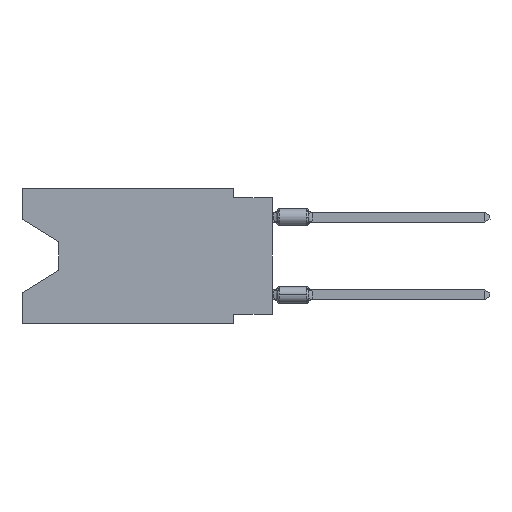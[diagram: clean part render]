
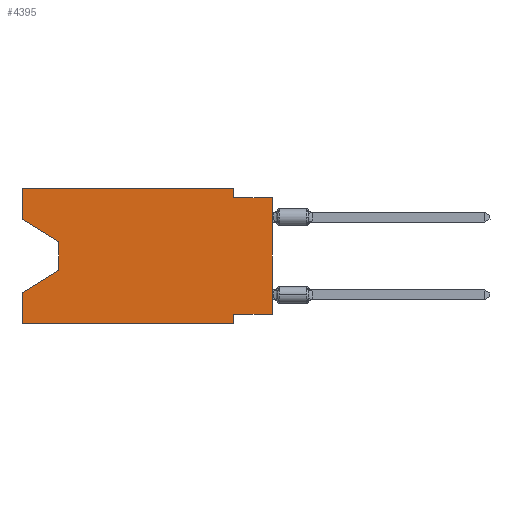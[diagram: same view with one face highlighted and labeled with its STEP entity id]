
A CAD part, left-side view. The second image highlights one B-rep face of the part: STEP entity #4395.
In plain terms, the highlighted planar face has unit normal (-1, 0, 0).
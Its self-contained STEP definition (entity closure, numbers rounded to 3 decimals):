
#636 = CARTESIAN_POINT ( 'NONE',  ( 0., 16.383, 0. ) ) ;
#758 = VERTEX_POINT ( 'NONE', #8095 ) ;
#846 = ORIENTED_EDGE ( 'NONE', *, *, #6919, .T. ) ;
#1065 = DIRECTION ( 'NONE',  ( 0., 0., -1. ) ) ;
#1217 = DIRECTION ( 'NONE',  ( 0., -0.855, -0.519 ) ) ;
#1262 = ORIENTED_EDGE ( 'NONE', *, *, #19110, .F. ) ;
#1602 = CARTESIAN_POINT ( 'NONE',  ( 0., 0., 0. ) ) ;
#1661 = ORIENTED_EDGE ( 'NONE', *, *, #12920, .F. ) ;
#2120 = DIRECTION ( 'NONE',  ( 0., -1., 0. ) ) ;
#2260 = CARTESIAN_POINT ( 'NONE',  ( 0., 2.54, 0. ) ) ;
#3335 = LINE ( 'NONE', #3458, #5462 ) ;
#3458 = CARTESIAN_POINT ( 'NONE',  ( 0., 16.383, 0. ) ) ;
#3691 = CARTESIAN_POINT ( 'NONE',  ( 0., 16.383, 0. ) ) ;
#3727 = LINE ( 'NONE', #21717, #14031 ) ;
#4017 = CARTESIAN_POINT ( 'NONE',  ( 0., 2.54, 0. ) ) ;
#4060 = CARTESIAN_POINT ( 'NONE',  ( 0., 16.383, 0. ) ) ;
#4395 = ADVANCED_FACE ( 'NONE', ( #16853 ), #10166, .F. ) ;
#4609 = EDGE_CURVE ( 'NONE', #20046, #12126, #15440, .T. ) ;
#4784 = CARTESIAN_POINT ( 'NONE',  ( 0., 2.54, -0.635 ) ) ;
#5031 = ORIENTED_EDGE ( 'NONE', *, *, #14738, .F. ) ;
#5048 = ORIENTED_EDGE ( 'NONE', *, *, #17432, .T. ) ;
#5152 = VERTEX_POINT ( 'NONE', #20845 ) ;
#5462 = VECTOR ( 'NONE', #10371, 1000. ) ;
#5563 = LINE ( 'NONE', #4060, #11293 ) ;
#5723 = EDGE_CURVE ( 'NONE', #17282, #21972, #11403, .T. ) ;
#5893 = LINE ( 'NONE', #12917, #9303 ) ;
#6027 = VECTOR ( 'NONE', #17652, 1000. ) ;
#6534 = VERTEX_POINT ( 'NONE', #636 ) ;
#6652 = CARTESIAN_POINT ( 'NONE',  ( 0., 0., -0.635 ) ) ;
#6772 = VECTOR ( 'NONE', #22127, 1000. ) ;
#6839 = CARTESIAN_POINT ( 'NONE',  ( 0., 16.383, -8.89 ) ) ;
#6886 = ORIENTED_EDGE ( 'NONE', *, *, #7499, .F. ) ;
#6919 = EDGE_CURVE ( 'NONE', #21859, #15292, #5893, .T. ) ;
#7285 = DIRECTION ( 'NONE',  ( 0., 0., -1. ) ) ;
#7499 = EDGE_CURVE ( 'NONE', #17193, #758, #7719, .T. ) ;
#7719 = LINE ( 'NONE', #6652, #15953 ) ;
#8095 = CARTESIAN_POINT ( 'NONE',  ( 0., 0., -0.635 ) ) ;
#8493 = DIRECTION ( 'NONE',  ( 0., -1., 0. ) ) ;
#8780 = CARTESIAN_POINT ( 'NONE',  ( 0., 16.383, -6.852 ) ) ;
#8879 = ORIENTED_EDGE ( 'NONE', *, *, #4609, .F. ) ;
#9303 = VECTOR ( 'NONE', #17780, 1000. ) ;
#9348 = LINE ( 'NONE', #11080, #10402 ) ;
#9779 = CARTESIAN_POINT ( 'NONE',  ( 0., 0., -8.255 ) ) ;
#10044 = DIRECTION ( 'NONE',  ( 1., 0., 0. ) ) ;
#10166 = PLANE ( 'NONE',  #11913 ) ;
#10371 = DIRECTION ( 'NONE',  ( 0., 0., 1. ) ) ;
#10402 = VECTOR ( 'NONE', #7285, 1000. ) ;
#10434 = LINE ( 'NONE', #15752, #20617 ) ;
#10548 = VECTOR ( 'NONE', #14482, 1000. ) ;
#11080 = CARTESIAN_POINT ( 'NONE',  ( 0., 2.54, -8.89 ) ) ;
#11215 = EDGE_CURVE ( 'NONE', #6534, #16757, #5563, .T. ) ;
#11293 = VECTOR ( 'NONE', #2120, 1000. ) ;
#11342 = ORIENTED_EDGE ( 'NONE', *, *, #14582, .T. ) ;
#11403 = LINE ( 'NONE', #16375, #13415 ) ;
#11913 = AXIS2_PLACEMENT_3D ( 'NONE', #18822, #10044, #1065 ) ;
#12126 = VERTEX_POINT ( 'NONE', #21549 ) ;
#12835 = CARTESIAN_POINT ( 'NONE',  ( 0., 0., -8.255 ) ) ;
#12917 = CARTESIAN_POINT ( 'NONE',  ( 0., 16.383, -8.89 ) ) ;
#12920 = EDGE_CURVE ( 'NONE', #5152, #6534, #3335, .T. ) ;
#13415 = VECTOR ( 'NONE', #21563, 1000. ) ;
#13595 = CARTESIAN_POINT ( 'NONE',  ( 0., 13.97, -3.505 ) ) ;
#13716 = EDGE_CURVE ( 'NONE', #5152, #14008, #10434, .T. ) ;
#14008 = VERTEX_POINT ( 'NONE', #13595 ) ;
#14031 = VECTOR ( 'NONE', #18141, 1000. ) ;
#14302 = LINE ( 'NONE', #3691, #6027 ) ;
#14482 = DIRECTION ( 'NONE',  ( 0., 0., -1. ) ) ;
#14582 = EDGE_CURVE ( 'NONE', #20046, #758, #17387, .T. ) ;
#14738 = EDGE_CURVE ( 'NONE', #16757, #17193, #18050, .T. ) ;
#14981 = ORIENTED_EDGE ( 'NONE', *, *, #11215, .F. ) ;
#15292 = VERTEX_POINT ( 'NONE', #21714 ) ;
#15440 = LINE ( 'NONE', #9779, #6772 ) ;
#15671 = DIRECTION ( 'NONE',  ( 0., 0., 1. ) ) ;
#15752 = CARTESIAN_POINT ( 'NONE',  ( 0., 16.383, -2.038 ) ) ;
#15953 = VECTOR ( 'NONE', #8493, 1000. ) ;
#16375 = CARTESIAN_POINT ( 'NONE',  ( 0., 13.97, -5.385 ) ) ;
#16757 = VERTEX_POINT ( 'NONE', #4017 ) ;
#16853 = FACE_OUTER_BOUND ( 'NONE', #22522, .T. ) ;
#17193 = VERTEX_POINT ( 'NONE', #4784 ) ;
#17282 = VERTEX_POINT ( 'NONE', #22096 ) ;
#17338 = ORIENTED_EDGE ( 'NONE', *, *, #20772, .F. ) ;
#17387 = LINE ( 'NONE', #1602, #19027 ) ;
#17432 = EDGE_CURVE ( 'NONE', #14008, #17282, #3727, .T. ) ;
#17652 = DIRECTION ( 'NONE',  ( 0., 0., 1. ) ) ;
#17780 = DIRECTION ( 'NONE',  ( 0., -1., 0. ) ) ;
#18050 = LINE ( 'NONE', #2260, #10548 ) ;
#18141 = DIRECTION ( 'NONE',  ( 0., 0., -1. ) ) ;
#18333 = ORIENTED_EDGE ( 'NONE', *, *, #5723, .T. ) ;
#18822 = CARTESIAN_POINT ( 'NONE',  ( 0., 16.383, 0. ) ) ;
#19027 = VECTOR ( 'NONE', #15671, 1000. ) ;
#19110 = EDGE_CURVE ( 'NONE', #12126, #15292, #9348, .T. ) ;
#20046 = VERTEX_POINT ( 'NONE', #12835 ) ;
#20267 = ORIENTED_EDGE ( 'NONE', *, *, #13716, .T. ) ;
#20617 = VECTOR ( 'NONE', #1217, 1000. ) ;
#20772 = EDGE_CURVE ( 'NONE', #21859, #21972, #14302, .T. ) ;
#20845 = CARTESIAN_POINT ( 'NONE',  ( 0., 16.383, -2.038 ) ) ;
#21549 = CARTESIAN_POINT ( 'NONE',  ( 0., 2.54, -8.255 ) ) ;
#21563 = DIRECTION ( 'NONE',  ( 0., 0.855, -0.519 ) ) ;
#21714 = CARTESIAN_POINT ( 'NONE',  ( 0., 2.54, -8.89 ) ) ;
#21717 = CARTESIAN_POINT ( 'NONE',  ( 0., 13.97, -3.505 ) ) ;
#21859 = VERTEX_POINT ( 'NONE', #6839 ) ;
#21972 = VERTEX_POINT ( 'NONE', #8780 ) ;
#22096 = CARTESIAN_POINT ( 'NONE',  ( 0., 13.97, -5.385 ) ) ;
#22127 = DIRECTION ( 'NONE',  ( 0., 1., 0. ) ) ;
#22522 = EDGE_LOOP ( 'NONE', ( #20267, #5048, #18333, #17338, #846, #1262, #8879, #11342, #6886, #5031, #14981, #1661 ) ) ;
